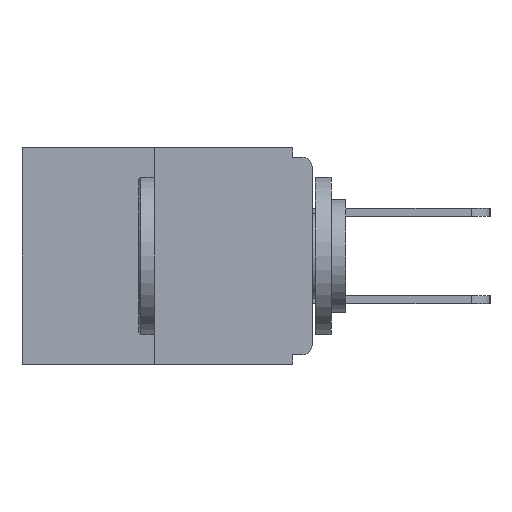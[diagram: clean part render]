
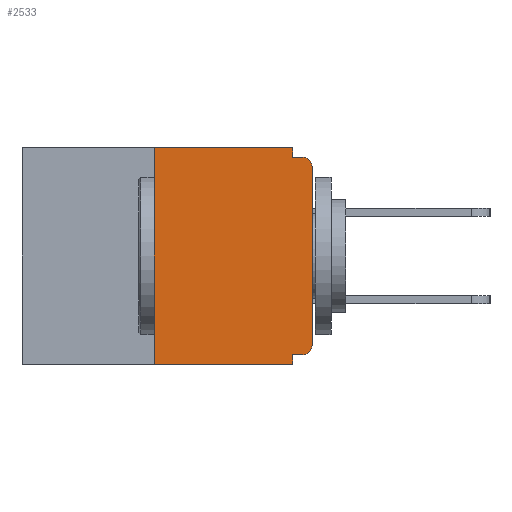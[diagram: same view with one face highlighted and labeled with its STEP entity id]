
A CAD part, left-side view. The second image highlights one B-rep face of the part: STEP entity #2533.
In plain terms, the highlighted planar face has unit normal (-1, 0, 0).
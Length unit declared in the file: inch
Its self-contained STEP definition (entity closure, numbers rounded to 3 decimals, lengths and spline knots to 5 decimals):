
#20 = CARTESIAN_POINT ( 'NONE',  ( 0., 0.015, -0.313 ) ) ;
#61 = LINE ( 'NONE', #12231, #2092 ) ;
#82 = LINE ( 'NONE', #9136, #10445 ) ;
#87 = DIRECTION ( 'NONE',  ( 0., 0., 1. ) ) ;
#112 = CIRCLE ( 'NONE', #10815, 0.015 ) ;
#348 = EDGE_CURVE ( 'NONE', #3902, #3551, #602, .T. ) ;
#367 = DIRECTION ( 'NONE',  ( 0., -1., 0. ) ) ;
#498 = VERTEX_POINT ( 'NONE', #2724 ) ;
#602 = LINE ( 'NONE', #10283, #12194 ) ;
#865 = EDGE_CURVE ( 'NONE', #3551, #1996, #61, .T. ) ;
#1335 = CARTESIAN_POINT ( 'NONE',  ( 0., 0.031, -0.015 ) ) ;
#1377 = PLANE ( 'NONE',  #3456 ) ;
#1677 = DIRECTION ( 'NONE',  ( 0., 1., 0. ) ) ;
#1752 = FACE_OUTER_BOUND ( 'NONE', #10366, .T. ) ;
#1996 = VERTEX_POINT ( 'NONE', #11739 ) ;
#2064 = CARTESIAN_POINT ( 'NONE',  ( 0., 0.015, -0.328 ) ) ;
#2092 = VECTOR ( 'NONE', #367, 39.37008 ) ;
#2512 = LINE ( 'NONE', #8866, #9102 ) ;
#2515 = CARTESIAN_POINT ( 'NONE',  ( 0., 0.031, -0.343 ) ) ;
#2533 = ADVANCED_FACE ( 'NONE', ( #1752 ), #1377, .F. ) ;
#2709 = VERTEX_POINT ( 'NONE', #4181 ) ;
#2724 = CARTESIAN_POINT ( 'NONE',  ( 0., 0.031, -0.328 ) ) ;
#2824 = ORIENTED_EDGE ( 'NONE', *, *, #8571, .F. ) ;
#2992 = LINE ( 'NONE', #5285, #11774 ) ;
#3027 = EDGE_CURVE ( 'NONE', #3902, #3109, #2992, .T. ) ;
#3109 = VERTEX_POINT ( 'NONE', #2515 ) ;
#3305 = VERTEX_POINT ( 'NONE', #12225 ) ;
#3398 = LINE ( 'NONE', #9068, #7803 ) ;
#3456 = AXIS2_PLACEMENT_3D ( 'NONE', #9536, #3562, #7430 ) ;
#3531 = CARTESIAN_POINT ( 'NONE',  ( 0., 0.25, -0.343 ) ) ;
#3551 = VERTEX_POINT ( 'NONE', #5925 ) ;
#3562 = DIRECTION ( 'NONE',  ( 1., 0., 0. ) ) ;
#3688 = AXIS2_PLACEMENT_3D ( 'NONE', #20, #3913, #12024 ) ;
#3733 = CARTESIAN_POINT ( 'NONE',  ( 0., 0., -0.328 ) ) ;
#3902 = VERTEX_POINT ( 'NONE', #3531 ) ;
#3913 = DIRECTION ( 'NONE',  ( -1., 0., 0. ) ) ;
#4181 = CARTESIAN_POINT ( 'NONE',  ( 0., 0., -0.03 ) ) ;
#4570 = ORIENTED_EDGE ( 'NONE', *, *, #7448, .T. ) ;
#4913 = VERTEX_POINT ( 'NONE', #1335 ) ;
#5090 = LINE ( 'NONE', #11762, #9965 ) ;
#5103 = ORIENTED_EDGE ( 'NONE', *, *, #865, .F. ) ;
#5285 = CARTESIAN_POINT ( 'NONE',  ( 0., 0.46, -0.343 ) ) ;
#5623 = ORIENTED_EDGE ( 'NONE', *, *, #12672, .F. ) ;
#5925 = CARTESIAN_POINT ( 'NONE',  ( 0., 0.25, 0. ) ) ;
#6173 = VERTEX_POINT ( 'NONE', #6753 ) ;
#6311 = EDGE_CURVE ( 'NONE', #3305, #2709, #3398, .T. ) ;
#6550 = EDGE_CURVE ( 'NONE', #2709, #6173, #112, .T. ) ;
#6558 = CARTESIAN_POINT ( 'NONE',  ( 0., 0.015, -0.03 ) ) ;
#6753 = CARTESIAN_POINT ( 'NONE',  ( 0., 0.015, -0.015 ) ) ;
#6757 = DIRECTION ( 'NONE',  ( 0., 0., -1. ) ) ;
#6883 = DIRECTION ( 'NONE',  ( 0., 0., -1. ) ) ;
#6967 = CIRCLE ( 'NONE', #3688, 0.015 ) ;
#7430 = DIRECTION ( 'NONE',  ( 0., 0., -1. ) ) ;
#7448 = EDGE_CURVE ( 'NONE', #11929, #3305, #6967, .T. ) ;
#7803 = VECTOR ( 'NONE', #87, 39.37008 ) ;
#7907 = EDGE_CURVE ( 'NONE', #4913, #6173, #82, .T. ) ;
#8472 = ORIENTED_EDGE ( 'NONE', *, *, #6550, .T. ) ;
#8571 = EDGE_CURVE ( 'NONE', #1996, #4913, #5090, .T. ) ;
#8866 = CARTESIAN_POINT ( 'NONE',  ( 0., 0.031, -0.343 ) ) ;
#8894 = VECTOR ( 'NONE', #1677, 39.37008 ) ;
#9058 = ORIENTED_EDGE ( 'NONE', *, *, #6311, .T. ) ;
#9068 = CARTESIAN_POINT ( 'NONE',  ( 0., 0., 0. ) ) ;
#9102 = VECTOR ( 'NONE', #6883, 39.37008 ) ;
#9136 = CARTESIAN_POINT ( 'NONE',  ( 0., 0., -0.015 ) ) ;
#9269 = DIRECTION ( 'NONE',  ( 0., -1., 0. ) ) ;
#9535 = LINE ( 'NONE', #3733, #8894 ) ;
#9536 = CARTESIAN_POINT ( 'NONE',  ( 0., 0.46, 0. ) ) ;
#9926 = ORIENTED_EDGE ( 'NONE', *, *, #3027, .T. ) ;
#9965 = VECTOR ( 'NONE', #6757, 39.37008 ) ;
#10283 = CARTESIAN_POINT ( 'NONE',  ( 0., 0.25, 0. ) ) ;
#10325 = DIRECTION ( 'NONE',  ( 0., -1., 0. ) ) ;
#10335 = ORIENTED_EDGE ( 'NONE', *, *, #7907, .F. ) ;
#10366 = EDGE_LOOP ( 'NONE', ( #5103, #11596, #9926, #10724, #5623, #4570, #9058, #8472, #10335, #2824 ) ) ;
#10440 = DIRECTION ( 'NONE',  ( -1., 0., 0. ) ) ;
#10445 = VECTOR ( 'NONE', #10325, 39.37008 ) ;
#10633 = EDGE_CURVE ( 'NONE', #498, #3109, #2512, .T. ) ;
#10724 = ORIENTED_EDGE ( 'NONE', *, *, #10633, .F. ) ;
#10815 = AXIS2_PLACEMENT_3D ( 'NONE', #6558, #10440, #12471 ) ;
#11596 = ORIENTED_EDGE ( 'NONE', *, *, #348, .F. ) ;
#11739 = CARTESIAN_POINT ( 'NONE',  ( 0., 0.031, 0. ) ) ;
#11762 = CARTESIAN_POINT ( 'NONE',  ( 0., 0.031, 0. ) ) ;
#11774 = VECTOR ( 'NONE', #9269, 39.37008 ) ;
#11929 = VERTEX_POINT ( 'NONE', #2064 ) ;
#12024 = DIRECTION ( 'NONE',  ( 0., 0., -1. ) ) ;
#12177 = DIRECTION ( 'NONE',  ( 0., 0., 1. ) ) ;
#12194 = VECTOR ( 'NONE', #12177, 39.37008 ) ;
#12225 = CARTESIAN_POINT ( 'NONE',  ( 0., 0., -0.313 ) ) ;
#12231 = CARTESIAN_POINT ( 'NONE',  ( 0., 0.46, 0. ) ) ;
#12471 = DIRECTION ( 'NONE',  ( 0., 0., -1. ) ) ;
#12672 = EDGE_CURVE ( 'NONE', #11929, #498, #9535, .T. ) ;
